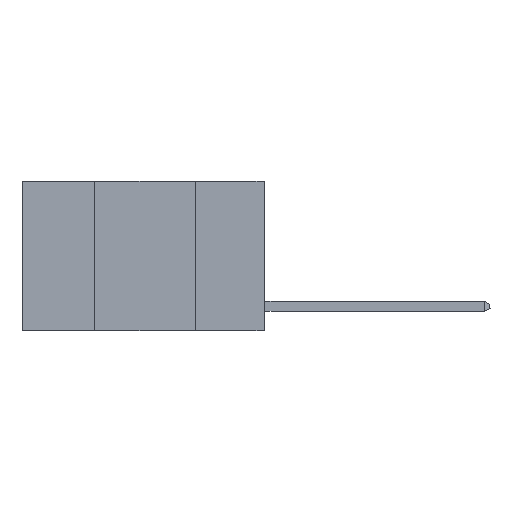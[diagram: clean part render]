
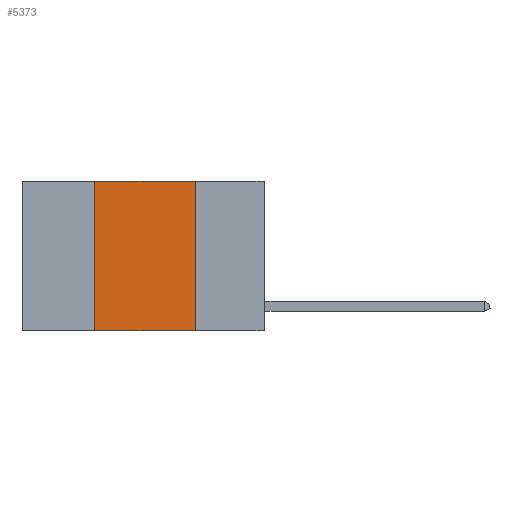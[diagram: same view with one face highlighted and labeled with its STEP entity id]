
A CAD part, left-side view. The second image highlights one B-rep face of the part: STEP entity #5373.
In plain terms, the highlighted planar face has unit normal (-1, 0, 0).
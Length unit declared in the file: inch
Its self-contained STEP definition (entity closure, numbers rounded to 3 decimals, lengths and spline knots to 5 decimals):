
#114 = VECTOR ( 'NONE', #1665, 39.37008 ) ;
#699 = VERTEX_POINT ( 'NONE', #3424 ) ;
#847 = ORIENTED_EDGE ( 'NONE', *, *, #2007, .F. ) ;
#961 = ORIENTED_EDGE ( 'NONE', *, *, #1044, .F. ) ;
#1044 = EDGE_CURVE ( 'NONE', #6745, #8860, #9042, .T. ) ;
#1665 = DIRECTION ( 'NONE',  ( 0., -1., 0. ) ) ;
#1816 = LINE ( 'NONE', #5936, #114 ) ;
#2007 = EDGE_CURVE ( 'NONE', #699, #6745, #10144, .T. ) ;
#2313 = LINE ( 'NONE', #2877, #8310 ) ;
#2758 = CARTESIAN_POINT ( 'NONE',  ( 0., 0.6, 0. ) ) ;
#2877 = CARTESIAN_POINT ( 'NONE',  ( 0., 0.42, 0. ) ) ;
#2907 = ORIENTED_EDGE ( 'NONE', *, *, #6573, .T. ) ;
#3248 = VECTOR ( 'NONE', #10955, 39.37008 ) ;
#3424 = CARTESIAN_POINT ( 'NONE',  ( 0., 0.42, 0. ) ) ;
#3587 = VERTEX_POINT ( 'NONE', #7241 ) ;
#4111 = DIRECTION ( 'NONE',  ( 0., 0., -1. ) ) ;
#4478 = CARTESIAN_POINT ( 'NONE',  ( 0., 0.17, 0. ) ) ;
#5233 = CARTESIAN_POINT ( 'NONE',  ( 0., 0.17, 0. ) ) ;
#5373 = ADVANCED_FACE ( 'NONE', ( #10593 ), #13832, .F. ) ;
#5936 = CARTESIAN_POINT ( 'NONE',  ( 0., 0.6, -0.37 ) ) ;
#6573 = EDGE_CURVE ( 'NONE', #3587, #8860, #1816, .T. ) ;
#6745 = VERTEX_POINT ( 'NONE', #5233 ) ;
#7076 = DIRECTION ( 'NONE',  ( 1., 0., 0. ) ) ;
#7241 = CARTESIAN_POINT ( 'NONE',  ( 0., 0.42, -0.37 ) ) ;
#8257 = CARTESIAN_POINT ( 'NONE',  ( 0., 0.6, 0. ) ) ;
#8310 = VECTOR ( 'NONE', #10361, 39.37008 ) ;
#8326 = ORIENTED_EDGE ( 'NONE', *, *, #11974, .F. ) ;
#8860 = VERTEX_POINT ( 'NONE', #14043 ) ;
#9042 = LINE ( 'NONE', #4478, #3248 ) ;
#10144 = LINE ( 'NONE', #8257, #11443 ) ;
#10361 = DIRECTION ( 'NONE',  ( 0., 0., 1. ) ) ;
#10593 = FACE_OUTER_BOUND ( 'NONE', #12941, .T. ) ;
#10955 = DIRECTION ( 'NONE',  ( 0., 0., -1. ) ) ;
#11443 = VECTOR ( 'NONE', #13306, 39.37008 ) ;
#11974 = EDGE_CURVE ( 'NONE', #3587, #699, #2313, .T. ) ;
#12609 = AXIS2_PLACEMENT_3D ( 'NONE', #2758, #7076, #4111 ) ;
#12941 = EDGE_LOOP ( 'NONE', ( #961, #847, #8326, #2907 ) ) ;
#13306 = DIRECTION ( 'NONE',  ( 0., -1., 0. ) ) ;
#13832 = PLANE ( 'NONE',  #12609 ) ;
#14043 = CARTESIAN_POINT ( 'NONE',  ( 0., 0.17, -0.37 ) ) ;
